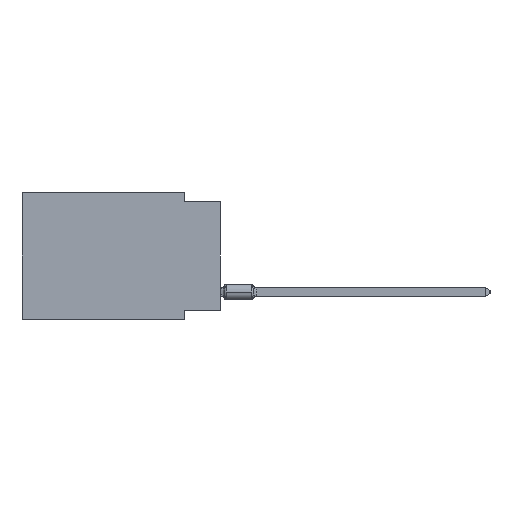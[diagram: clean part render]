
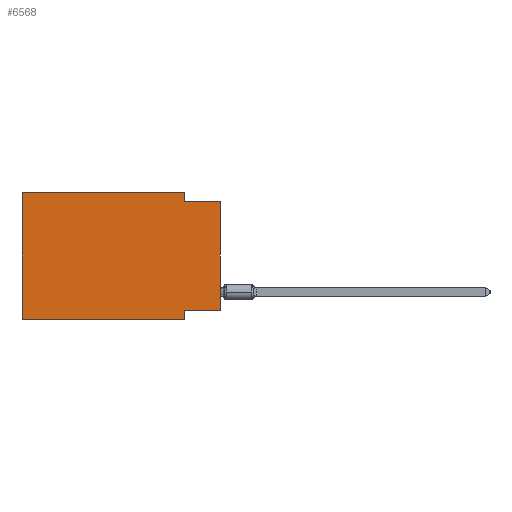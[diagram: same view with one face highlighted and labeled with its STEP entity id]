
A CAD part, left-side view. The second image highlights one B-rep face of the part: STEP entity #6568.
In plain terms, the highlighted planar face has unit normal (-1, 0, 0).
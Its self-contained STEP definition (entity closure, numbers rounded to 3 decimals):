
#204 = AXIS2_PLACEMENT_3D ( 'NONE', #23450, #8144, #19559 ) ;
#546 = VECTOR ( 'NONE', #1001, 1000. ) ;
#586 = LINE ( 'NONE', #11758, #20149 ) ;
#715 = DIRECTION ( 'NONE',  ( 0., 0., -1. ) ) ;
#1001 = DIRECTION ( 'NONE',  ( 0., 0., 1. ) ) ;
#1160 = EDGE_CURVE ( 'NONE', #11491, #2190, #17518, .T. ) ;
#1543 = DIRECTION ( 'NONE',  ( 0., 0., 1. ) ) ;
#1586 = VECTOR ( 'NONE', #715, 1000. ) ;
#1629 = DIRECTION ( 'NONE',  ( 0., -1., 0. ) ) ;
#2090 = CARTESIAN_POINT ( 'NONE',  ( 0., 0., -8.255 ) ) ;
#2190 = VERTEX_POINT ( 'NONE', #21803 ) ;
#2890 = ORIENTED_EDGE ( 'NONE', *, *, #16494, .F. ) ;
#3360 = CARTESIAN_POINT ( 'NONE',  ( 0., 13.97, 0. ) ) ;
#3842 = CARTESIAN_POINT ( 'NONE',  ( 0., 0., -0.635 ) ) ;
#4095 = CARTESIAN_POINT ( 'NONE',  ( 0., 2.54, 0. ) ) ;
#4118 = VERTEX_POINT ( 'NONE', #18198 ) ;
#5177 = VERTEX_POINT ( 'NONE', #8356 ) ;
#5231 = VERTEX_POINT ( 'NONE', #12757 ) ;
#5331 = CARTESIAN_POINT ( 'NONE',  ( 0., 13.97, -8.89 ) ) ;
#5718 = EDGE_LOOP ( 'NONE', ( #16297, #22804, #21512, #2890, #7140, #15535, #16022, #17299 ) ) ;
#6568 = ADVANCED_FACE ( 'NONE', ( #12067 ), #15973, .F. ) ;
#7140 = ORIENTED_EDGE ( 'NONE', *, *, #13755, .F. ) ;
#7596 = DIRECTION ( 'NONE',  ( 0., -1., 0. ) ) ;
#7660 = EDGE_CURVE ( 'NONE', #2190, #12864, #20881, .T. ) ;
#8144 = DIRECTION ( 'NONE',  ( 1., 0., 0. ) ) ;
#8261 = CARTESIAN_POINT ( 'NONE',  ( 0., 0., 0. ) ) ;
#8356 = CARTESIAN_POINT ( 'NONE',  ( 0., 13.97, 0. ) ) ;
#9143 = LINE ( 'NONE', #3360, #17761 ) ;
#9358 = EDGE_CURVE ( 'NONE', #13733, #23513, #586, .T. ) ;
#10041 = CARTESIAN_POINT ( 'NONE',  ( 0., 2.54, 0. ) ) ;
#10973 = VECTOR ( 'NONE', #17834, 1000. ) ;
#11491 = VERTEX_POINT ( 'NONE', #4095 ) ;
#11758 = CARTESIAN_POINT ( 'NONE',  ( 0., 13.97, -8.89 ) ) ;
#12067 = FACE_OUTER_BOUND ( 'NONE', #5718, .T. ) ;
#12404 = EDGE_CURVE ( 'NONE', #4118, #23513, #14032, .T. ) ;
#12757 = CARTESIAN_POINT ( 'NONE',  ( 0., 0., -8.255 ) ) ;
#12863 = CARTESIAN_POINT ( 'NONE',  ( 0., 0., -0.635 ) ) ;
#12864 = VERTEX_POINT ( 'NONE', #12863 ) ;
#13733 = VERTEX_POINT ( 'NONE', #5331 ) ;
#13755 = EDGE_CURVE ( 'NONE', #13733, #5177, #9143, .T. ) ;
#13985 = EDGE_CURVE ( 'NONE', #5231, #12864, #14132, .T. ) ;
#14032 = LINE ( 'NONE', #15988, #10973 ) ;
#14054 = VECTOR ( 'NONE', #19270, 1000. ) ;
#14132 = LINE ( 'NONE', #8261, #546 ) ;
#15535 = ORIENTED_EDGE ( 'NONE', *, *, #9358, .T. ) ;
#15973 = PLANE ( 'NONE',  #204 ) ;
#15988 = CARTESIAN_POINT ( 'NONE',  ( 0., 2.54, -8.89 ) ) ;
#16022 = ORIENTED_EDGE ( 'NONE', *, *, #12404, .F. ) ;
#16297 = ORIENTED_EDGE ( 'NONE', *, *, #13985, .T. ) ;
#16494 = EDGE_CURVE ( 'NONE', #5177, #11491, #21069, .T. ) ;
#16574 = CARTESIAN_POINT ( 'NONE',  ( 0., 13.97, 0. ) ) ;
#17042 = LINE ( 'NONE', #2090, #14054 ) ;
#17206 = DIRECTION ( 'NONE',  ( 0., -1., 0. ) ) ;
#17299 = ORIENTED_EDGE ( 'NONE', *, *, #19268, .F. ) ;
#17518 = LINE ( 'NONE', #10041, #1586 ) ;
#17761 = VECTOR ( 'NONE', #1543, 1000. ) ;
#17834 = DIRECTION ( 'NONE',  ( 0., 0., -1. ) ) ;
#18198 = CARTESIAN_POINT ( 'NONE',  ( 0., 2.54, -8.255 ) ) ;
#19268 = EDGE_CURVE ( 'NONE', #5231, #4118, #17042, .T. ) ;
#19270 = DIRECTION ( 'NONE',  ( 0., 1., 0. ) ) ;
#19559 = DIRECTION ( 'NONE',  ( 0., 0., -1. ) ) ;
#20149 = VECTOR ( 'NONE', #7596, 1000. ) ;
#20881 = LINE ( 'NONE', #3842, #22572 ) ;
#21069 = LINE ( 'NONE', #16574, #21848 ) ;
#21512 = ORIENTED_EDGE ( 'NONE', *, *, #1160, .F. ) ;
#21803 = CARTESIAN_POINT ( 'NONE',  ( 0., 2.54, -0.635 ) ) ;
#21848 = VECTOR ( 'NONE', #1629, 1000. ) ;
#22572 = VECTOR ( 'NONE', #17206, 1000. ) ;
#22731 = CARTESIAN_POINT ( 'NONE',  ( 0., 2.54, -8.89 ) ) ;
#22804 = ORIENTED_EDGE ( 'NONE', *, *, #7660, .F. ) ;
#23450 = CARTESIAN_POINT ( 'NONE',  ( 0., 13.97, 0. ) ) ;
#23513 = VERTEX_POINT ( 'NONE', #22731 ) ;
